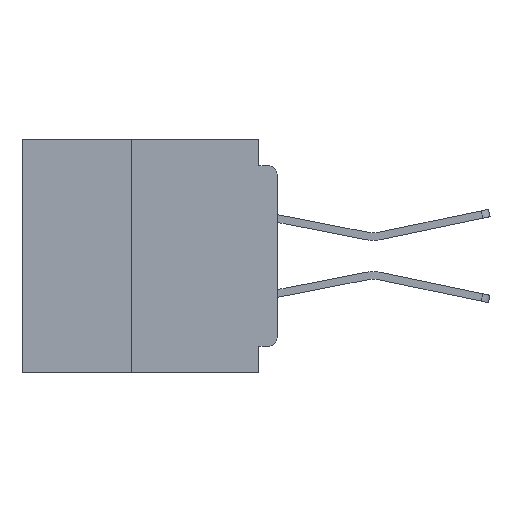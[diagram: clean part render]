
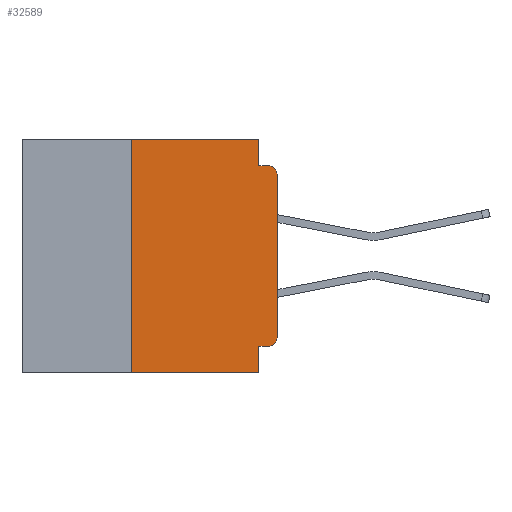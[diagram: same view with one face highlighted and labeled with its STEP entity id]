
A CAD part, left-side view. The second image highlights one B-rep face of the part: STEP entity #32589.
In plain terms, the highlighted planar face has unit normal (-1, 0, 0).
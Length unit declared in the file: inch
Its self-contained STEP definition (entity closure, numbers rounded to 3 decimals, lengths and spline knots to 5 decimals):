
#64 = DIRECTION ( 'NONE',  ( -1., 0., 0. ) ) ;
#312 = VERTEX_POINT ( 'NONE', #24170 ) ;
#471 = ORIENTED_EDGE ( 'NONE', *, *, #27655, .F. ) ;
#711 = VERTEX_POINT ( 'NONE', #17114 ) ;
#1721 = CIRCLE ( 'NONE', #5955, 0.015 ) ;
#2454 = VECTOR ( 'NONE', #45755, 39.37008 ) ;
#2675 = EDGE_CURVE ( 'NONE', #26331, #52047, #8788, .T. ) ;
#2910 = CIRCLE ( 'NONE', #15278, 0.015 ) ;
#3388 = VECTOR ( 'NONE', #5193, 39.37008 ) ;
#3419 = ORIENTED_EDGE ( 'NONE', *, *, #46980, .F. ) ;
#3864 = LINE ( 'NONE', #9859, #2454 ) ;
#4266 = CARTESIAN_POINT ( 'NONE',  ( 0., 0.031, -0.4 ) ) ;
#4681 = FACE_OUTER_BOUND ( 'NONE', #20289, .T. ) ;
#5193 = DIRECTION ( 'NONE',  ( 0., 1., 0. ) ) ;
#5259 = DIRECTION ( 'NONE',  ( 0., 0., -1. ) ) ;
#5955 = AXIS2_PLACEMENT_3D ( 'NONE', #26844, #64, #31375 ) ;
#6790 = VERTEX_POINT ( 'NONE', #4266 ) ;
#7491 = ORIENTED_EDGE ( 'NONE', *, *, #2675, .F. ) ;
#7562 = ORIENTED_EDGE ( 'NONE', *, *, #52966, .F. ) ;
#8759 = LINE ( 'NONE', #25607, #31214 ) ;
#8788 = LINE ( 'NONE', #29186, #19301 ) ;
#9754 = CARTESIAN_POINT ( 'NONE',  ( 0., 0.015, -0.06 ) ) ;
#9859 = CARTESIAN_POINT ( 'NONE',  ( 0., 0.031, 0. ) ) ;
#9933 = LINE ( 'NONE', #39251, #21879 ) ;
#12168 = VERTEX_POINT ( 'NONE', #50167 ) ;
#14234 = DIRECTION ( 'NONE',  ( 0., 0., -1. ) ) ;
#15278 = AXIS2_PLACEMENT_3D ( 'NONE', #9754, #41118, #14234 ) ;
#16536 = CARTESIAN_POINT ( 'NONE',  ( 0., 0.25, -0.4 ) ) ;
#17114 = CARTESIAN_POINT ( 'NONE',  ( 0., 0., -0.06 ) ) ;
#17588 = EDGE_CURVE ( 'NONE', #711, #36390, #2910, .T. ) ;
#18637 = ORIENTED_EDGE ( 'NONE', *, *, #39989, .T. ) ;
#19301 = VECTOR ( 'NONE', #28346, 39.37008 ) ;
#20289 = EDGE_LOOP ( 'NONE', ( #49373, #42410, #38365, #7562, #7491, #471, #51497, #52382, #3419, #18637 ) ) ;
#21879 = VECTOR ( 'NONE', #43776, 39.37008 ) ;
#22209 = EDGE_CURVE ( 'NONE', #52076, #6790, #49986, .T. ) ;
#22946 = CARTESIAN_POINT ( 'NONE',  ( 0., 0., -0.355 ) ) ;
#23940 = EDGE_CURVE ( 'NONE', #57027, #711, #9933, .T. ) ;
#24170 = CARTESIAN_POINT ( 'NONE',  ( 0., 0.031, -0.045 ) ) ;
#25607 = CARTESIAN_POINT ( 'NONE',  ( 0., 0.031, -0.4 ) ) ;
#26331 = VERTEX_POINT ( 'NONE', #38620 ) ;
#26844 = CARTESIAN_POINT ( 'NONE',  ( 0., 0.015, -0.34 ) ) ;
#27521 = CARTESIAN_POINT ( 'NONE',  ( 0., 0.437, 0. ) ) ;
#27638 = EDGE_CURVE ( 'NONE', #48426, #6790, #8759, .T. ) ;
#27655 = EDGE_CURVE ( 'NONE', #52076, #26331, #54907, .T. ) ;
#27662 = EDGE_CURVE ( 'NONE', #312, #36390, #53515, .T. ) ;
#28346 = DIRECTION ( 'NONE',  ( 0., -1., 0. ) ) ;
#29012 = VECTOR ( 'NONE', #53631, 39.37008 ) ;
#29186 = CARTESIAN_POINT ( 'NONE',  ( 0., 0.437, 0. ) ) ;
#29971 = LINE ( 'NONE', #22946, #3388 ) ;
#30136 = DIRECTION ( 'NONE',  ( 0., 0., -1. ) ) ;
#30338 = DIRECTION ( 'NONE',  ( 0., -1., 0. ) ) ;
#31214 = VECTOR ( 'NONE', #30136, 39.37008 ) ;
#31375 = DIRECTION ( 'NONE',  ( 0., 0., -1. ) ) ;
#32034 = DIRECTION ( 'NONE',  ( 1., 0., 0. ) ) ;
#32589 = ADVANCED_FACE ( 'NONE', ( #4681 ), #54244, .F. ) ;
#34660 = CARTESIAN_POINT ( 'NONE',  ( 0., 0., -0.045 ) ) ;
#36390 = VERTEX_POINT ( 'NONE', #50260 ) ;
#38365 = ORIENTED_EDGE ( 'NONE', *, *, #27662, .F. ) ;
#38620 = CARTESIAN_POINT ( 'NONE',  ( 0., 0.25, 0. ) ) ;
#39251 = CARTESIAN_POINT ( 'NONE',  ( 0., 0., 0. ) ) ;
#39989 = EDGE_CURVE ( 'NONE', #12168, #57027, #1721, .T. ) ;
#40283 = VECTOR ( 'NONE', #30338, 39.37008 ) ;
#41118 = DIRECTION ( 'NONE',  ( -1., 0., 0. ) ) ;
#41706 = VECTOR ( 'NONE', #52366, 39.37008 ) ;
#42410 = ORIENTED_EDGE ( 'NONE', *, *, #17588, .T. ) ;
#43776 = DIRECTION ( 'NONE',  ( 0., 0., 1. ) ) ;
#44107 = CARTESIAN_POINT ( 'NONE',  ( 0., 0., -0.34 ) ) ;
#44323 = CARTESIAN_POINT ( 'NONE',  ( 0., 0.031, -0.355 ) ) ;
#44760 = CARTESIAN_POINT ( 'NONE',  ( 0., 0.437, -0.4 ) ) ;
#45755 = DIRECTION ( 'NONE',  ( 0., 0., -1. ) ) ;
#46980 = EDGE_CURVE ( 'NONE', #12168, #48426, #29971, .T. ) ;
#47945 = CARTESIAN_POINT ( 'NONE',  ( 0., 0.031, 0. ) ) ;
#48426 = VERTEX_POINT ( 'NONE', #44323 ) ;
#48969 = AXIS2_PLACEMENT_3D ( 'NONE', #27521, #32034, #5259 ) ;
#49373 = ORIENTED_EDGE ( 'NONE', *, *, #23940, .T. ) ;
#49986 = LINE ( 'NONE', #44760, #29012 ) ;
#50167 = CARTESIAN_POINT ( 'NONE',  ( 0., 0.015, -0.355 ) ) ;
#50260 = CARTESIAN_POINT ( 'NONE',  ( 0., 0.015, -0.045 ) ) ;
#51497 = ORIENTED_EDGE ( 'NONE', *, *, #22209, .T. ) ;
#52047 = VERTEX_POINT ( 'NONE', #47945 ) ;
#52076 = VERTEX_POINT ( 'NONE', #57158 ) ;
#52366 = DIRECTION ( 'NONE',  ( 0., 0., 1. ) ) ;
#52382 = ORIENTED_EDGE ( 'NONE', *, *, #27638, .F. ) ;
#52966 = EDGE_CURVE ( 'NONE', #52047, #312, #3864, .T. ) ;
#53515 = LINE ( 'NONE', #34660, #40283 ) ;
#53631 = DIRECTION ( 'NONE',  ( 0., -1., 0. ) ) ;
#54244 = PLANE ( 'NONE',  #48969 ) ;
#54907 = LINE ( 'NONE', #16536, #41706 ) ;
#57027 = VERTEX_POINT ( 'NONE', #44107 ) ;
#57158 = CARTESIAN_POINT ( 'NONE',  ( 0., 0.25, -0.4 ) ) ;
